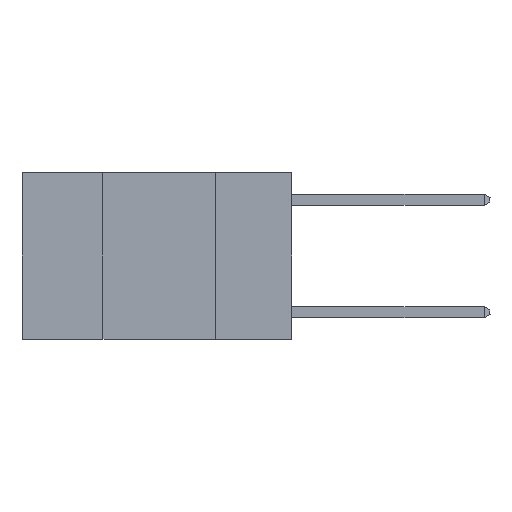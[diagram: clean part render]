
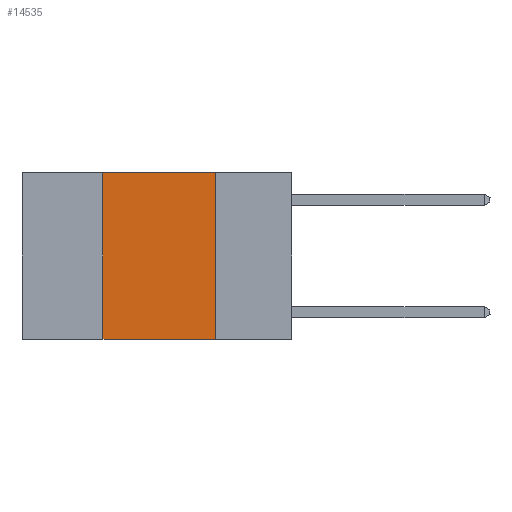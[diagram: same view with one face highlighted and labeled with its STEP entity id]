
A CAD part, left-side view. The second image highlights one B-rep face of the part: STEP entity #14535.
In plain terms, the highlighted planar face has unit normal (-1, 0, 0).
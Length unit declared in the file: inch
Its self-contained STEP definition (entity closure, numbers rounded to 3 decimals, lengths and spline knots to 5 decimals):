
#981 = ORIENTED_EDGE ( 'NONE', *, *, #15413, .T. ) ;
#1729 = FACE_OUTER_BOUND ( 'NONE', #13741, .T. ) ;
#2006 = VERTEX_POINT ( 'NONE', #13490 ) ;
#2188 = LINE ( 'NONE', #14644, #14230 ) ;
#2405 = VERTEX_POINT ( 'NONE', #12431 ) ;
#3141 = LINE ( 'NONE', #13182, #3727 ) ;
#3257 = CARTESIAN_POINT ( 'NONE',  ( 0., 0.6, 0. ) ) ;
#3682 = CARTESIAN_POINT ( 'NONE',  ( 0., 0.42, 0. ) ) ;
#3727 = VECTOR ( 'NONE', #11975, 39.37008 ) ;
#5198 = ORIENTED_EDGE ( 'NONE', *, *, #12003, .F. ) ;
#5382 = ORIENTED_EDGE ( 'NONE', *, *, #10761, .F. ) ;
#5693 = DIRECTION ( 'NONE',  ( 0., -1., 0. ) ) ;
#5882 = VERTEX_POINT ( 'NONE', #3682 ) ;
#5888 = DIRECTION ( 'NONE',  ( 0., 0., -1. ) ) ;
#5938 = VERTEX_POINT ( 'NONE', #14996 ) ;
#6993 = DIRECTION ( 'NONE',  ( 0., 0., 1. ) ) ;
#7112 = AXIS2_PLACEMENT_3D ( 'NONE', #8368, #14513, #5888 ) ;
#8368 = CARTESIAN_POINT ( 'NONE',  ( 0., 0.6, 0. ) ) ;
#8616 = VECTOR ( 'NONE', #5693, 39.37008 ) ;
#8775 = ORIENTED_EDGE ( 'NONE', *, *, #13569, .F. ) ;
#9215 = CARTESIAN_POINT ( 'NONE',  ( 0., 0.42, 0. ) ) ;
#10761 = EDGE_CURVE ( 'NONE', #5882, #2006, #14408, .T. ) ;
#11823 = LINE ( 'NONE', #9215, #15145 ) ;
#11975 = DIRECTION ( 'NONE',  ( 0., -1., 0. ) ) ;
#12003 = EDGE_CURVE ( 'NONE', #2006, #5938, #2188, .T. ) ;
#12431 = CARTESIAN_POINT ( 'NONE',  ( 0., 0.42, -0.37 ) ) ;
#12997 = PLANE ( 'NONE',  #7112 ) ;
#13182 = CARTESIAN_POINT ( 'NONE',  ( 0., 0.6, -0.37 ) ) ;
#13490 = CARTESIAN_POINT ( 'NONE',  ( 0., 0.17, 0. ) ) ;
#13569 = EDGE_CURVE ( 'NONE', #2405, #5882, #11823, .T. ) ;
#13741 = EDGE_LOOP ( 'NONE', ( #5198, #5382, #8775, #981 ) ) ;
#14230 = VECTOR ( 'NONE', #15959, 39.37008 ) ;
#14408 = LINE ( 'NONE', #3257, #8616 ) ;
#14513 = DIRECTION ( 'NONE',  ( 1., 0., 0. ) ) ;
#14535 = ADVANCED_FACE ( 'NONE', ( #1729 ), #12997, .F. ) ;
#14644 = CARTESIAN_POINT ( 'NONE',  ( 0., 0.17, 0. ) ) ;
#14996 = CARTESIAN_POINT ( 'NONE',  ( 0., 0.17, -0.37 ) ) ;
#15145 = VECTOR ( 'NONE', #6993, 39.37008 ) ;
#15413 = EDGE_CURVE ( 'NONE', #2405, #5938, #3141, .T. ) ;
#15959 = DIRECTION ( 'NONE',  ( 0., 0., -1. ) ) ;
